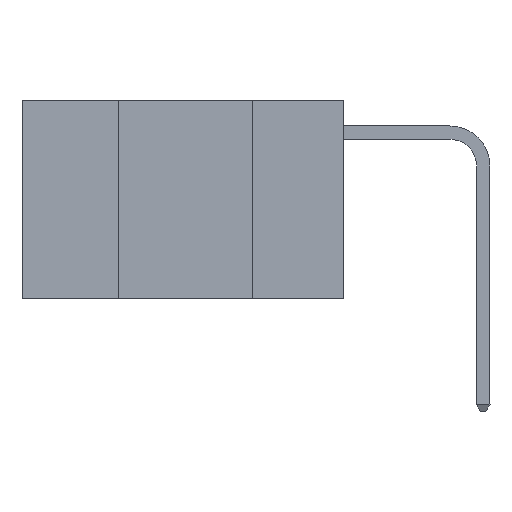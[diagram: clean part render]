
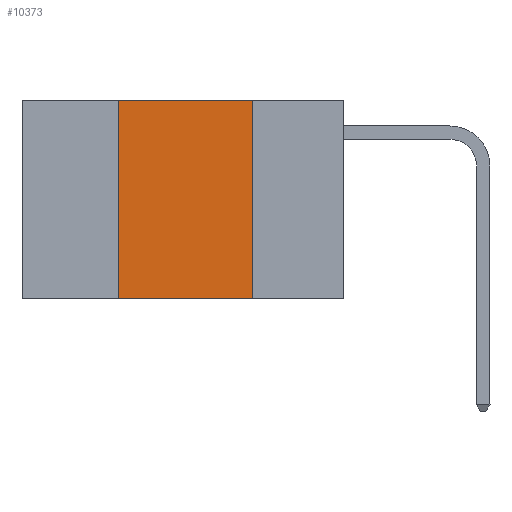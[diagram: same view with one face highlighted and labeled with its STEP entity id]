
A CAD part, left-side view. The second image highlights one B-rep face of the part: STEP entity #10373.
In plain terms, the highlighted planar face has unit normal (-1, 0, 0).
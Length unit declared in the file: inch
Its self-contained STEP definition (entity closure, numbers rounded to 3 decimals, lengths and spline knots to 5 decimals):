
#105 = EDGE_CURVE ( 'NONE', #24741, #21994, #18469, .T. ) ;
#2985 = LINE ( 'NONE', #22379, #21207 ) ;
#3104 = DIRECTION ( 'NONE',  ( 0., 0., -1. ) ) ;
#5095 = PLANE ( 'NONE',  #15872 ) ;
#5694 = CARTESIAN_POINT ( 'NONE',  ( 0., 0.17, 0. ) ) ;
#6791 = VECTOR ( 'NONE', #22958, 39.37008 ) ;
#6927 = CARTESIAN_POINT ( 'NONE',  ( 0., 0.17, 0. ) ) ;
#9438 = EDGE_LOOP ( 'NONE', ( #16437, #11499, #13944, #10849 ) ) ;
#10373 = ADVANCED_FACE ( 'NONE', ( #18374 ), #5095, .F. ) ;
#10849 = ORIENTED_EDGE ( 'NONE', *, *, #105, .T. ) ;
#11105 = DIRECTION ( 'NONE',  ( 1., 0., 0. ) ) ;
#11260 = LINE ( 'NONE', #11382, #23802 ) ;
#11382 = CARTESIAN_POINT ( 'NONE',  ( 0., 0.42, 0. ) ) ;
#11499 = ORIENTED_EDGE ( 'NONE', *, *, #19506, .F. ) ;
#11687 = VERTEX_POINT ( 'NONE', #23886 ) ;
#13944 = ORIENTED_EDGE ( 'NONE', *, *, #24334, .F. ) ;
#14171 = CARTESIAN_POINT ( 'NONE',  ( 0., 0.17, -0.37 ) ) ;
#14710 = CARTESIAN_POINT ( 'NONE',  ( 0., 0.6, -0.37 ) ) ;
#15872 = AXIS2_PLACEMENT_3D ( 'NONE', #16868, #11105, #3104 ) ;
#16437 = ORIENTED_EDGE ( 'NONE', *, *, #21393, .F. ) ;
#16485 = VERTEX_POINT ( 'NONE', #6927 ) ;
#16868 = CARTESIAN_POINT ( 'NONE',  ( 0., 0.6, 0. ) ) ;
#17391 = DIRECTION ( 'NONE',  ( 0., 0., 1. ) ) ;
#18235 = DIRECTION ( 'NONE',  ( 0., -1., 0. ) ) ;
#18374 = FACE_OUTER_BOUND ( 'NONE', #9438, .T. ) ;
#18469 = LINE ( 'NONE', #14710, #23549 ) ;
#19506 = EDGE_CURVE ( 'NONE', #11687, #16485, #2985, .T. ) ;
#21207 = VECTOR ( 'NONE', #23997, 39.37008 ) ;
#21393 = EDGE_CURVE ( 'NONE', #16485, #21994, #22839, .T. ) ;
#21994 = VERTEX_POINT ( 'NONE', #14171 ) ;
#22379 = CARTESIAN_POINT ( 'NONE',  ( 0., 0.6, 0. ) ) ;
#22380 = CARTESIAN_POINT ( 'NONE',  ( 0., 0.42, -0.37 ) ) ;
#22839 = LINE ( 'NONE', #5694, #6791 ) ;
#22958 = DIRECTION ( 'NONE',  ( 0., 0., -1. ) ) ;
#23549 = VECTOR ( 'NONE', #18235, 39.37008 ) ;
#23802 = VECTOR ( 'NONE', #17391, 39.37008 ) ;
#23886 = CARTESIAN_POINT ( 'NONE',  ( 0., 0.42, 0. ) ) ;
#23997 = DIRECTION ( 'NONE',  ( 0., -1., 0. ) ) ;
#24334 = EDGE_CURVE ( 'NONE', #24741, #11687, #11260, .T. ) ;
#24741 = VERTEX_POINT ( 'NONE', #22380 ) ;
